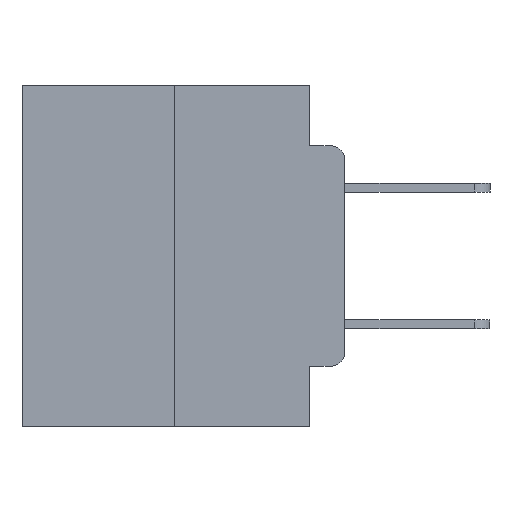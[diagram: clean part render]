
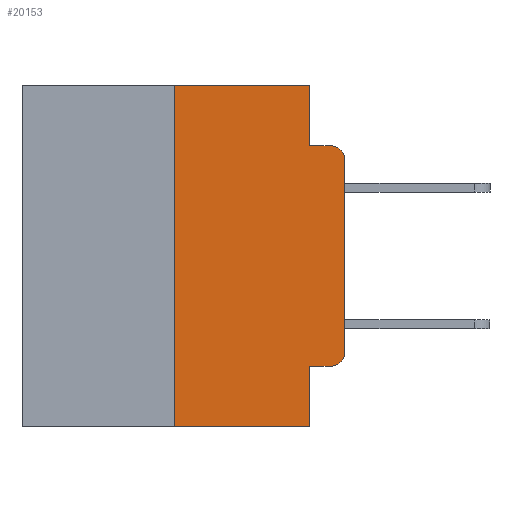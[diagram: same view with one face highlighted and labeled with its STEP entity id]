
A CAD part, left-side view. The second image highlights one B-rep face of the part: STEP entity #20153.
In plain terms, the highlighted planar face has unit normal (-1, 0, 0).
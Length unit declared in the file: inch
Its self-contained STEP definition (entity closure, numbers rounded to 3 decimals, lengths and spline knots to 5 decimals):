
#156 = VERTEX_POINT ( 'NONE', #25130 ) ;
#1166 = VERTEX_POINT ( 'NONE', #8128 ) ;
#1327 = DIRECTION ( 'NONE',  ( 0., 0., -1. ) ) ;
#1641 = DIRECTION ( 'NONE',  ( 0., 0., -1. ) ) ;
#1780 = LINE ( 'NONE', #21606, #6716 ) ;
#1974 = CARTESIAN_POINT ( 'NONE',  ( 0., 0.25, -0.5 ) ) ;
#2051 = CARTESIAN_POINT ( 'NONE',  ( 0., 0.473, 0. ) ) ;
#2061 = ORIENTED_EDGE ( 'NONE', *, *, #6948, .F. ) ;
#2106 = CARTESIAN_POINT ( 'NONE',  ( 0., 0.051, -0.0885 ) ) ;
#3512 = FACE_OUTER_BOUND ( 'NONE', #11764, .T. ) ;
#3578 = VECTOR ( 'NONE', #22204, 39.37008 ) ;
#4196 = DIRECTION ( 'NONE',  ( 0., -1., 0. ) ) ;
#4436 = LINE ( 'NONE', #20486, #8646 ) ;
#5013 = DIRECTION ( 'NONE',  ( 0., -1., 0. ) ) ;
#5093 = VERTEX_POINT ( 'NONE', #10120 ) ;
#5457 = CIRCLE ( 'NONE', #13144, 0.02 ) ;
#6519 = DIRECTION ( 'NONE',  ( 0., 0., -1. ) ) ;
#6716 = VECTOR ( 'NONE', #7672, 39.37008 ) ;
#6948 = EDGE_CURVE ( 'NONE', #10423, #18321, #1780, .T. ) ;
#7105 = LINE ( 'NONE', #19132, #16448 ) ;
#7464 = LINE ( 'NONE', #20993, #8086 ) ;
#7672 = DIRECTION ( 'NONE',  ( 0., 0., -1. ) ) ;
#7918 = CARTESIAN_POINT ( 'NONE',  ( 0., 0.051, -0.0885 ) ) ;
#8077 = ORIENTED_EDGE ( 'NONE', *, *, #19957, .T. ) ;
#8086 = VECTOR ( 'NONE', #9041, 39.37008 ) ;
#8128 = CARTESIAN_POINT ( 'NONE',  ( 0., 0.25, 0. ) ) ;
#8616 = AXIS2_PLACEMENT_3D ( 'NONE', #11637, #13591, #1327 ) ;
#8646 = VECTOR ( 'NONE', #6519, 39.37008 ) ;
#9041 = DIRECTION ( 'NONE',  ( 0., 0., 1. ) ) ;
#9354 = VERTEX_POINT ( 'NONE', #19199 ) ;
#9659 = EDGE_CURVE ( 'NONE', #10839, #1166, #22083, .T. ) ;
#10120 = CARTESIAN_POINT ( 'NONE',  ( 0., 0.02, -0.0885 ) ) ;
#10166 = EDGE_CURVE ( 'NONE', #19013, #156, #5457, .T. ) ;
#10423 = VERTEX_POINT ( 'NONE', #22576 ) ;
#10615 = ORIENTED_EDGE ( 'NONE', *, *, #20821, .F. ) ;
#10839 = VERTEX_POINT ( 'NONE', #1974 ) ;
#11403 = CARTESIAN_POINT ( 'NONE',  ( 0., 0.02, -0.1085 ) ) ;
#11565 = VECTOR ( 'NONE', #24188, 39.37008 ) ;
#11595 = CARTESIAN_POINT ( 'NONE',  ( 0., 0.051, -0.4115 ) ) ;
#11637 = CARTESIAN_POINT ( 'NONE',  ( 0., 0.473, 0. ) ) ;
#11764 = EDGE_LOOP ( 'NONE', ( #8077, #14004, #16496, #2061, #19275, #15270, #19899, #10615, #19455, #13581 ) ) ;
#11891 = VERTEX_POINT ( 'NONE', #11595 ) ;
#12838 = LINE ( 'NONE', #2106, #18086 ) ;
#13144 = AXIS2_PLACEMENT_3D ( 'NONE', #25812, #13875, #1641 ) ;
#13177 = LINE ( 'NONE', #2051, #23164 ) ;
#13369 = DIRECTION ( 'NONE',  ( 0., 0., -1. ) ) ;
#13581 = ORIENTED_EDGE ( 'NONE', *, *, #10166, .T. ) ;
#13591 = DIRECTION ( 'NONE',  ( 1., 0., 0. ) ) ;
#13875 = DIRECTION ( 'NONE',  ( -1., 0., 0. ) ) ;
#14004 = ORIENTED_EDGE ( 'NONE', *, *, #22931, .T. ) ;
#14267 = DIRECTION ( 'NONE',  ( 0., -1., 0. ) ) ;
#14720 = EDGE_CURVE ( 'NONE', #10839, #25225, #24983, .T. ) ;
#15138 = CARTESIAN_POINT ( 'NONE',  ( 0., 0.051, -0.5 ) ) ;
#15270 = ORIENTED_EDGE ( 'NONE', *, *, #9659, .F. ) ;
#15815 = CARTESIAN_POINT ( 'NONE',  ( 0., 0.473, -0.5 ) ) ;
#16448 = VECTOR ( 'NONE', #5013, 39.37008 ) ;
#16496 = ORIENTED_EDGE ( 'NONE', *, *, #19108, .F. ) ;
#17957 = CARTESIAN_POINT ( 'NONE',  ( 0., 0.02, -0.4115 ) ) ;
#18086 = VECTOR ( 'NONE', #4196, 39.37008 ) ;
#18321 = VERTEX_POINT ( 'NONE', #7918 ) ;
#18458 = EDGE_CURVE ( 'NONE', #1166, #10423, #13177, .T. ) ;
#19013 = VERTEX_POINT ( 'NONE', #17957 ) ;
#19108 = EDGE_CURVE ( 'NONE', #18321, #5093, #12838, .T. ) ;
#19132 = CARTESIAN_POINT ( 'NONE',  ( 0., 0.051, -0.4115 ) ) ;
#19199 = CARTESIAN_POINT ( 'NONE',  ( 0., 0., -0.1085 ) ) ;
#19275 = ORIENTED_EDGE ( 'NONE', *, *, #18458, .F. ) ;
#19325 = AXIS2_PLACEMENT_3D ( 'NONE', #11403, #25300, #13369 ) ;
#19455 = ORIENTED_EDGE ( 'NONE', *, *, #23536, .T. ) ;
#19899 = ORIENTED_EDGE ( 'NONE', *, *, #14720, .T. ) ;
#19957 = EDGE_CURVE ( 'NONE', #156, #9354, #7464, .T. ) ;
#20153 = ADVANCED_FACE ( 'NONE', ( #3512 ), #23543, .F. ) ;
#20486 = CARTESIAN_POINT ( 'NONE',  ( 0., 0.051, 0. ) ) ;
#20821 = EDGE_CURVE ( 'NONE', #11891, #25225, #4436, .T. ) ;
#20993 = CARTESIAN_POINT ( 'NONE',  ( 0., 0., 0. ) ) ;
#21606 = CARTESIAN_POINT ( 'NONE',  ( 0., 0.051, 0. ) ) ;
#22083 = LINE ( 'NONE', #22167, #11565 ) ;
#22167 = CARTESIAN_POINT ( 'NONE',  ( 0., 0.25, 0. ) ) ;
#22204 = DIRECTION ( 'NONE',  ( 0., -1., 0. ) ) ;
#22576 = CARTESIAN_POINT ( 'NONE',  ( 0., 0.051, 0. ) ) ;
#22931 = EDGE_CURVE ( 'NONE', #9354, #5093, #25544, .T. ) ;
#23164 = VECTOR ( 'NONE', #14267, 39.37008 ) ;
#23536 = EDGE_CURVE ( 'NONE', #11891, #19013, #7105, .T. ) ;
#23543 = PLANE ( 'NONE',  #8616 ) ;
#24188 = DIRECTION ( 'NONE',  ( 0., 0., 1. ) ) ;
#24983 = LINE ( 'NONE', #15815, #3578 ) ;
#25130 = CARTESIAN_POINT ( 'NONE',  ( 0., 0., -0.3915 ) ) ;
#25225 = VERTEX_POINT ( 'NONE', #15138 ) ;
#25300 = DIRECTION ( 'NONE',  ( -1., 0., 0. ) ) ;
#25544 = CIRCLE ( 'NONE', #19325, 0.02 ) ;
#25812 = CARTESIAN_POINT ( 'NONE',  ( 0., 0.02, -0.3915 ) ) ;
